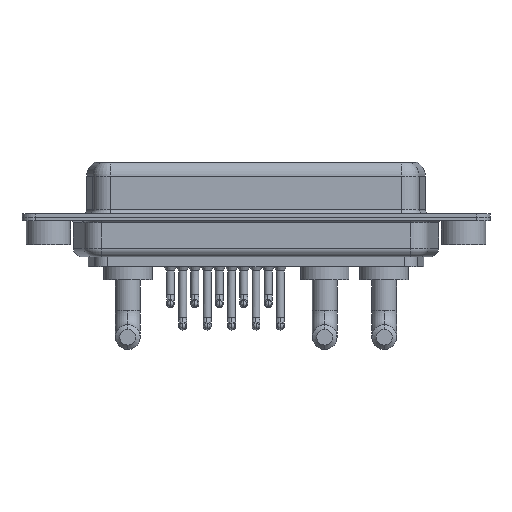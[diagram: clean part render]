
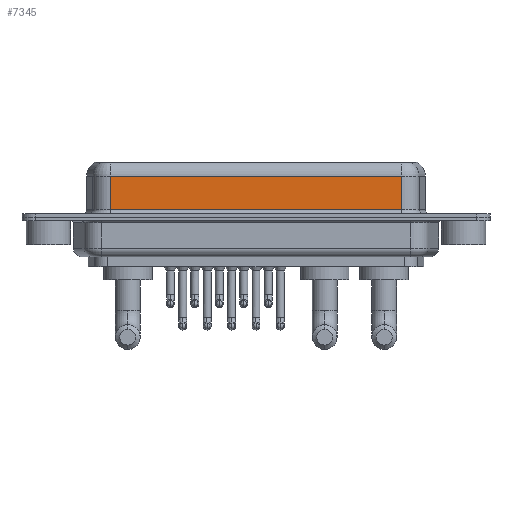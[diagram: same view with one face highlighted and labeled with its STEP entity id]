
A CAD part, front view. The second image highlights one B-rep face of the part: STEP entity #7345.
In plain terms, the highlighted planar face has unit normal (0, -1, 0).
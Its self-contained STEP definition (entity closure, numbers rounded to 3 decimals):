
#267 = CARTESIAN_POINT ( 'NONE',  ( 40.037, -3.95, 6.4 ) ) ;
#391 = CARTESIAN_POINT ( 'NONE',  ( 7.013, -3.95, 6.4 ) ) ;
#486 = LINE ( 'NONE', #391, #7057 ) ;
#567 = EDGE_CURVE ( 'NONE', #14303, #1540, #5115, .T. ) ;
#850 = VECTOR ( 'NONE', #6449, 1000. ) ;
#1540 = VERTEX_POINT ( 'NONE', #14833 ) ;
#1943 = DIRECTION ( 'NONE',  ( -1., 0., 0. ) ) ;
#2129 = DIRECTION ( 'NONE',  ( 0., 0., -1. ) ) ;
#2568 = EDGE_CURVE ( 'NONE', #15113, #15263, #15390, .T. ) ;
#4887 = DIRECTION ( 'NONE',  ( 0., 0., 1. ) ) ;
#4985 = CARTESIAN_POINT ( 'NONE',  ( 40.037, -3.95, 6.4 ) ) ;
#5115 = LINE ( 'NONE', #16748, #9951 ) ;
#6237 = EDGE_CURVE ( 'NONE', #14303, #15263, #7130, .T. ) ;
#6449 = DIRECTION ( 'NONE',  ( 1., 0., 0. ) ) ;
#6450 = CARTESIAN_POINT ( 'NONE',  ( 40.037, -3.95, 0.9 ) ) ;
#7057 = VECTOR ( 'NONE', #2129, 1000. ) ;
#7130 = LINE ( 'NONE', #267, #9824 ) ;
#7345 = ADVANCED_FACE ( 'NONE', ( #9200 ), #12171, .F. ) ;
#7581 = DIRECTION ( 'NONE',  ( 0., 0., -1. ) ) ;
#9200 = FACE_OUTER_BOUND ( 'NONE', #13560, .T. ) ;
#9824 = VECTOR ( 'NONE', #7581, 1000. ) ;
#9951 = VECTOR ( 'NONE', #1943, 1000. ) ;
#11043 = EDGE_CURVE ( 'NONE', #1540, #15113, #486, .T. ) ;
#11077 = CARTESIAN_POINT ( 'NONE',  ( 7.013, -3.95, 0.9 ) ) ;
#12171 = PLANE ( 'NONE',  #17834 ) ;
#12939 = ORIENTED_EDGE ( 'NONE', *, *, #567, .T. ) ;
#13560 = EDGE_LOOP ( 'NONE', ( #15563, #12939, #14686, #17058 ) ) ;
#14303 = VERTEX_POINT ( 'NONE', #16977 ) ;
#14686 = ORIENTED_EDGE ( 'NONE', *, *, #11043, .T. ) ;
#14833 = CARTESIAN_POINT ( 'NONE',  ( 7.013, -3.95, 4.65 ) ) ;
#15113 = VERTEX_POINT ( 'NONE', #11077 ) ;
#15263 = VERTEX_POINT ( 'NONE', #6450 ) ;
#15390 = LINE ( 'NONE', #16535, #850 ) ;
#15563 = ORIENTED_EDGE ( 'NONE', *, *, #6237, .F. ) ;
#16535 = CARTESIAN_POINT ( 'NONE',  ( 40.037, -3.95, 0.9 ) ) ;
#16748 = CARTESIAN_POINT ( 'NONE',  ( 40.037, -3.95, 4.65 ) ) ;
#16977 = CARTESIAN_POINT ( 'NONE',  ( 40.037, -3.95, 4.65 ) ) ;
#17058 = ORIENTED_EDGE ( 'NONE', *, *, #2568, .T. ) ;
#17834 = AXIS2_PLACEMENT_3D ( 'NONE', #4985, #18071, #4887 ) ;
#18071 = DIRECTION ( 'NONE',  ( 0., 1., 0. ) ) ;
